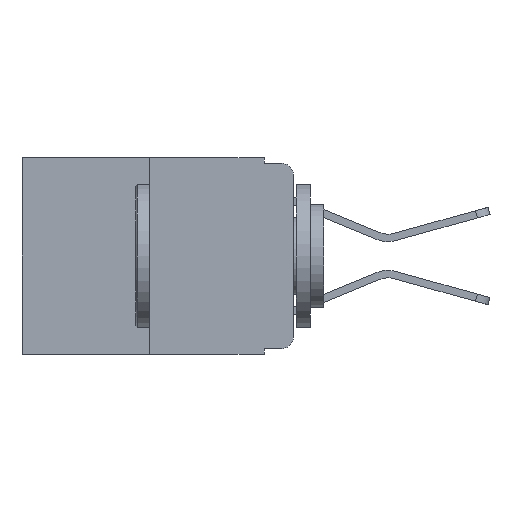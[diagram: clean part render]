
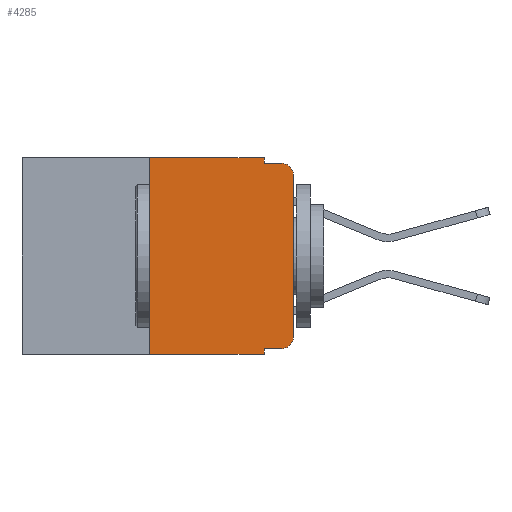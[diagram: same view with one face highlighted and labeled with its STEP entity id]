
A CAD part, left-side view. The second image highlights one B-rep face of the part: STEP entity #4285.
In plain terms, the highlighted planar face has unit normal (-1, 0, 0).
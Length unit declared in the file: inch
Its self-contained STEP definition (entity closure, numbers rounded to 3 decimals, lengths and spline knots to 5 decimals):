
#294 = EDGE_CURVE ( 'NONE', #16371, #356, #18288, .T. ) ;
#356 = VERTEX_POINT ( 'NONE', #5886 ) ;
#505 = FACE_OUTER_BOUND ( 'NONE', #9522, .T. ) ;
#620 = CARTESIAN_POINT ( 'NONE',  ( 0., 0.02, -0.03 ) ) ;
#897 = DIRECTION ( 'NONE',  ( -1., 0., 0. ) ) ;
#1224 = VECTOR ( 'NONE', #4194, 39.37008 ) ;
#1736 = ORIENTED_EDGE ( 'NONE', *, *, #22649, .F. ) ;
#2117 = CARTESIAN_POINT ( 'NONE',  ( 0., 0.051, -0.01 ) ) ;
#2178 = CARTESIAN_POINT ( 'NONE',  ( 0., 0.02, -0.01 ) ) ;
#2521 = ORIENTED_EDGE ( 'NONE', *, *, #15370, .F. ) ;
#2582 = CARTESIAN_POINT ( 'NONE',  ( 0., 0.051, -0.01 ) ) ;
#2684 = VECTOR ( 'NONE', #3564, 39.37008 ) ;
#3014 = CIRCLE ( 'NONE', #18234, 0.02 ) ;
#3564 = DIRECTION ( 'NONE',  ( 0., 0., -1. ) ) ;
#3671 = VERTEX_POINT ( 'NONE', #10634 ) ;
#3764 = CARTESIAN_POINT ( 'NONE',  ( 0., 0.051, -0.333 ) ) ;
#4026 = EDGE_CURVE ( 'NONE', #24571, #18568, #24639, .T. ) ;
#4118 = LINE ( 'NONE', #12396, #4398 ) ;
#4194 = DIRECTION ( 'NONE',  ( 0., -1., 0. ) ) ;
#4285 = ADVANCED_FACE ( 'NONE', ( #505 ), #7192, .F. ) ;
#4398 = VECTOR ( 'NONE', #6395, 39.37008 ) ;
#5154 = DIRECTION ( 'NONE',  ( 0., 0., -1. ) ) ;
#5558 = CARTESIAN_POINT ( 'NONE',  ( 0., 0., -0.313 ) ) ;
#5886 = CARTESIAN_POINT ( 'NONE',  ( 0., 0.25, 0. ) ) ;
#6373 = VERTEX_POINT ( 'NONE', #2178 ) ;
#6395 = DIRECTION ( 'NONE',  ( 0., 0., -1. ) ) ;
#7058 = CARTESIAN_POINT ( 'NONE',  ( 0., 0.473, 0. ) ) ;
#7192 = PLANE ( 'NONE',  #19690 ) ;
#8126 = CARTESIAN_POINT ( 'NONE',  ( 0., 0.473, 0. ) ) ;
#8135 = AXIS2_PLACEMENT_3D ( 'NONE', #620, #25687, #14808 ) ;
#8986 = VECTOR ( 'NONE', #12789, 39.37008 ) ;
#9522 = EDGE_LOOP ( 'NONE', ( #16053, #23720, #2521, #23866, #1736, #18217, #12952, #26731, #10544, #12208 ) ) ;
#9677 = CARTESIAN_POINT ( 'NONE',  ( 0., 0.25, 0. ) ) ;
#10459 = VECTOR ( 'NONE', #23836, 39.37008 ) ;
#10544 = ORIENTED_EDGE ( 'NONE', *, *, #15812, .T. ) ;
#10634 = CARTESIAN_POINT ( 'NONE',  ( 0., 0., -0.03 ) ) ;
#10702 = DIRECTION ( 'NONE',  ( 0., -1., 0. ) ) ;
#11258 = CARTESIAN_POINT ( 'NONE',  ( 0., 0.02, -0.313 ) ) ;
#11316 = CARTESIAN_POINT ( 'NONE',  ( 0., 0., 0. ) ) ;
#11751 = CARTESIAN_POINT ( 'NONE',  ( 0., 0.02, -0.333 ) ) ;
#11856 = LINE ( 'NONE', #11316, #18379 ) ;
#12208 = ORIENTED_EDGE ( 'NONE', *, *, #17186, .T. ) ;
#12334 = VERTEX_POINT ( 'NONE', #23410 ) ;
#12396 = CARTESIAN_POINT ( 'NONE',  ( 0., 0.051, 0. ) ) ;
#12439 = VERTEX_POINT ( 'NONE', #5558 ) ;
#12789 = DIRECTION ( 'NONE',  ( 0., -1., 0. ) ) ;
#12913 = CIRCLE ( 'NONE', #8135, 0.02 ) ;
#12952 = ORIENTED_EDGE ( 'NONE', *, *, #24962, .T. ) ;
#14808 = DIRECTION ( 'NONE',  ( 0., 0., -1. ) ) ;
#15370 = EDGE_CURVE ( 'NONE', #18568, #6373, #23243, .T. ) ;
#15384 = DIRECTION ( 'NONE',  ( 0., 0., -1. ) ) ;
#15517 = DIRECTION ( 'NONE',  ( 1., 0., 0. ) ) ;
#15801 = EDGE_CURVE ( 'NONE', #3671, #6373, #12913, .T. ) ;
#15812 = EDGE_CURVE ( 'NONE', #21488, #18847, #21271, .T. ) ;
#16053 = ORIENTED_EDGE ( 'NONE', *, *, #26024, .T. ) ;
#16371 = VERTEX_POINT ( 'NONE', #26432 ) ;
#17186 = EDGE_CURVE ( 'NONE', #18847, #12439, #3014, .T. ) ;
#17613 = DIRECTION ( 'NONE',  ( 0., 0., 1. ) ) ;
#18217 = ORIENTED_EDGE ( 'NONE', *, *, #294, .F. ) ;
#18234 = AXIS2_PLACEMENT_3D ( 'NONE', #11258, #897, #5154 ) ;
#18288 = LINE ( 'NONE', #9677, #24561 ) ;
#18379 = VECTOR ( 'NONE', #17613, 39.37008 ) ;
#18568 = VERTEX_POINT ( 'NONE', #2117 ) ;
#18847 = VERTEX_POINT ( 'NONE', #11751 ) ;
#19690 = AXIS2_PLACEMENT_3D ( 'NONE', #7058, #15517, #15384 ) ;
#20409 = CARTESIAN_POINT ( 'NONE',  ( 0., 0.051, 0. ) ) ;
#21271 = LINE ( 'NONE', #21554, #23469 ) ;
#21347 = LINE ( 'NONE', #25761, #10459 ) ;
#21488 = VERTEX_POINT ( 'NONE', #3764 ) ;
#21554 = CARTESIAN_POINT ( 'NONE',  ( 0., 0.051, -0.333 ) ) ;
#22649 = EDGE_CURVE ( 'NONE', #356, #24571, #26921, .T. ) ;
#23243 = LINE ( 'NONE', #2582, #8986 ) ;
#23410 = CARTESIAN_POINT ( 'NONE',  ( 0., 0.051, -0.343 ) ) ;
#23469 = VECTOR ( 'NONE', #10702, 39.37008 ) ;
#23720 = ORIENTED_EDGE ( 'NONE', *, *, #15801, .T. ) ;
#23836 = DIRECTION ( 'NONE',  ( 0., -1., 0. ) ) ;
#23866 = ORIENTED_EDGE ( 'NONE', *, *, #4026, .F. ) ;
#24358 = CARTESIAN_POINT ( 'NONE',  ( 0., 0.051, 0. ) ) ;
#24561 = VECTOR ( 'NONE', #26843, 39.37008 ) ;
#24571 = VERTEX_POINT ( 'NONE', #20409 ) ;
#24639 = LINE ( 'NONE', #24358, #2684 ) ;
#24962 = EDGE_CURVE ( 'NONE', #16371, #12334, #21347, .T. ) ;
#25209 = EDGE_CURVE ( 'NONE', #21488, #12334, #4118, .T. ) ;
#25687 = DIRECTION ( 'NONE',  ( -1., 0., 0. ) ) ;
#25761 = CARTESIAN_POINT ( 'NONE',  ( 0., 0.473, -0.343 ) ) ;
#26024 = EDGE_CURVE ( 'NONE', #12439, #3671, #11856, .T. ) ;
#26432 = CARTESIAN_POINT ( 'NONE',  ( 0., 0.25, -0.343 ) ) ;
#26731 = ORIENTED_EDGE ( 'NONE', *, *, #25209, .F. ) ;
#26843 = DIRECTION ( 'NONE',  ( 0., 0., 1. ) ) ;
#26921 = LINE ( 'NONE', #8126, #1224 ) ;
